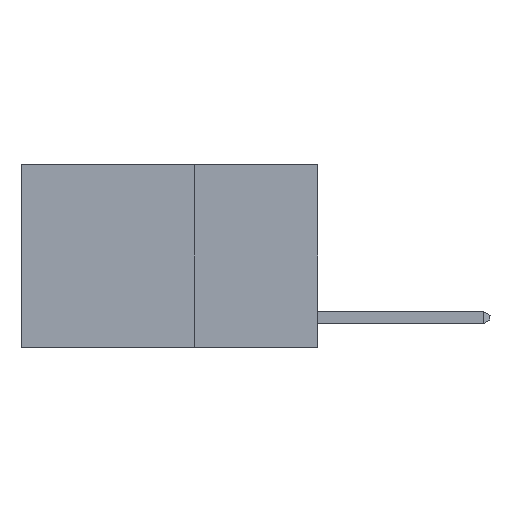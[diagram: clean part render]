
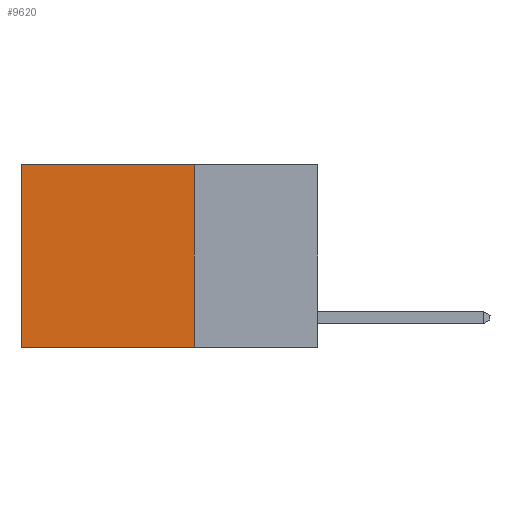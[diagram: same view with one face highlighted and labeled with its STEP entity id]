
A CAD part, left-side view. The second image highlights one B-rep face of the part: STEP entity #9620.
In plain terms, the highlighted planar face has unit normal (-1, 0, 0).
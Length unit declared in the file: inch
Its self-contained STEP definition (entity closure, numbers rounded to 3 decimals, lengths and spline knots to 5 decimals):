
#224 = ORIENTED_EDGE ( 'NONE', *, *, #8120, .T. ) ;
#513 = VERTEX_POINT ( 'NONE', #613 ) ;
#530 = ORIENTED_EDGE ( 'NONE', *, *, #7769, .F. ) ;
#613 = CARTESIAN_POINT ( 'NONE',  ( 0.2625, 0.6, -0.37 ) ) ;
#731 = ORIENTED_EDGE ( 'NONE', *, *, #11564, .F. ) ;
#1019 = CARTESIAN_POINT ( 'NONE',  ( 0.2625, 0.6, 0. ) ) ;
#1454 = VERTEX_POINT ( 'NONE', #6238 ) ;
#1802 = VECTOR ( 'NONE', #7228, 39.37008 ) ;
#2222 = CARTESIAN_POINT ( 'NONE',  ( 0.2625, 0.25, -0.37 ) ) ;
#2396 = DIRECTION ( 'NONE',  ( 1., 0., 0. ) ) ;
#2935 = AXIS2_PLACEMENT_3D ( 'NONE', #8109, #2396, #9047 ) ;
#2989 = LINE ( 'NONE', #9186, #10834 ) ;
#3560 = DIRECTION ( 'NONE',  ( 0., 1., 0. ) ) ;
#4350 = VERTEX_POINT ( 'NONE', #8499 ) ;
#4354 = LINE ( 'NONE', #1019, #11586 ) ;
#5312 = EDGE_CURVE ( 'NONE', #1454, #4350, #6918, .T. ) ;
#5628 = VECTOR ( 'NONE', #6668, 39.37008 ) ;
#6238 = CARTESIAN_POINT ( 'NONE',  ( 0.2625, 0.25, 0. ) ) ;
#6668 = DIRECTION ( 'NONE',  ( 0., 0., -1. ) ) ;
#6918 = LINE ( 'NONE', #8468, #1802 ) ;
#7055 = VERTEX_POINT ( 'NONE', #2222 ) ;
#7228 = DIRECTION ( 'NONE',  ( 0., 1., 0. ) ) ;
#7269 = EDGE_LOOP ( 'NONE', ( #224, #530, #731, #7718 ) ) ;
#7542 = LINE ( 'NONE', #12330, #5628 ) ;
#7718 = ORIENTED_EDGE ( 'NONE', *, *, #5312, .T. ) ;
#7769 = EDGE_CURVE ( 'NONE', #7055, #513, #2989, .T. ) ;
#8109 = CARTESIAN_POINT ( 'NONE',  ( 0.2625, 0.25, 0. ) ) ;
#8120 = EDGE_CURVE ( 'NONE', #4350, #513, #4354, .T. ) ;
#8468 = CARTESIAN_POINT ( 'NONE',  ( 0.2625, 0.25, 0. ) ) ;
#8499 = CARTESIAN_POINT ( 'NONE',  ( 0.2625, 0.6, 0. ) ) ;
#9047 = DIRECTION ( 'NONE',  ( 0., 0., -1. ) ) ;
#9150 = FACE_OUTER_BOUND ( 'NONE', #7269, .T. ) ;
#9186 = CARTESIAN_POINT ( 'NONE',  ( 0.2625, 0.25, -0.37 ) ) ;
#9620 = ADVANCED_FACE ( 'NONE', ( #9150 ), #11891, .F. ) ;
#10618 = DIRECTION ( 'NONE',  ( 0., 0., -1. ) ) ;
#10834 = VECTOR ( 'NONE', #3560, 39.37008 ) ;
#11564 = EDGE_CURVE ( 'NONE', #1454, #7055, #7542, .T. ) ;
#11586 = VECTOR ( 'NONE', #10618, 39.37008 ) ;
#11891 = PLANE ( 'NONE',  #2935 ) ;
#12330 = CARTESIAN_POINT ( 'NONE',  ( 0.2625, 0.25, 0. ) ) ;
